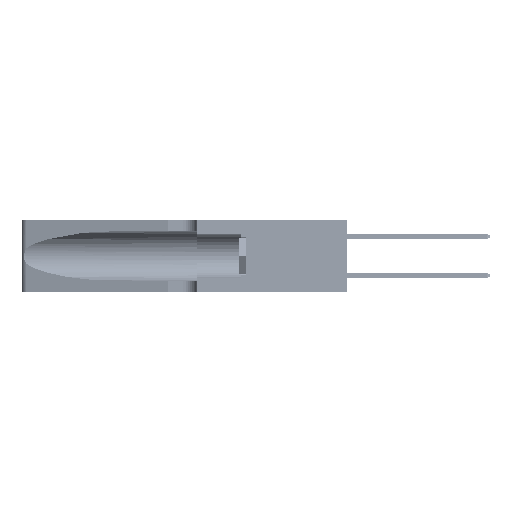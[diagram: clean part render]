
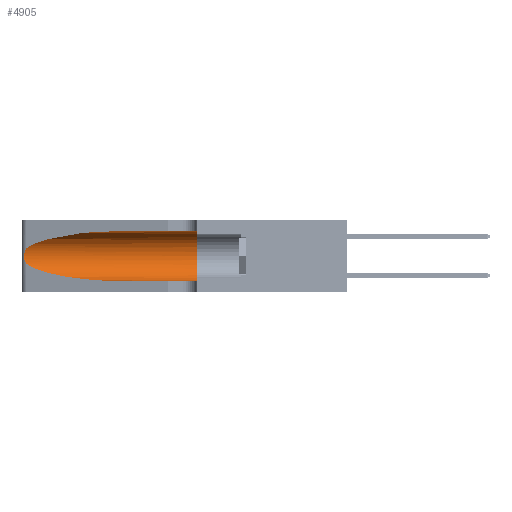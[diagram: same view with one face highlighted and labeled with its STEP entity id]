
A CAD part, left-side view. The second image highlights one B-rep face of the part: STEP entity #4905.
In plain terms, the highlighted cylindrical face has radius 3.308 mm (diameter 6.617 mm), a partial arc.
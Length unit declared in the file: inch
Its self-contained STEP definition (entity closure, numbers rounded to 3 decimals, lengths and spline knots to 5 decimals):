
#337 =( BOUNDED_CURVE ( )  B_SPLINE_CURVE ( 3, ( #11936, #41555, #20118, #29381 ),
 .UNSPECIFIED., .F., .F. ) 
 B_SPLINE_CURVE_WITH_KNOTS ( ( 4, 4 ),
 ( 3.44316, 4.71239 ),
 .UNSPECIFIED. ) 
 CURVE ( )  GEOMETRIC_REPRESENTATION_ITEM ( )  RATIONAL_B_SPLINE_CURVE ( ( 1., 0.87, 0.87, 1. ) ) 
 REPRESENTATION_ITEM ( '' )  );
#1661 = LINE ( 'NONE', #37860, #40006 ) ;
#2851 = CARTESIAN_POINT ( 'NONE',  ( 0.25639, 1.23184, 0.21858 ) ) ;
#2947 = EDGE_CURVE ( 'NONE', #52856, #15381, #337, .T. ) ;
#4281 = VERTEX_POINT ( 'NONE', #29657 ) ;
#4905 = ADVANCED_FACE ( 'NONE', ( #43117 ), #30594, .F. ) ;
#5707 = ORIENTED_EDGE ( 'NONE', *, *, #17141, .T. ) ;
#6196 = ORIENTED_EDGE ( 'NONE', *, *, #31475, .T. ) ;
#6332 = EDGE_CURVE ( 'NONE', #4281, #52856, #23085, .T. ) ;
#6570 = CARTESIAN_POINT ( 'NONE',  ( 0.25856, 1.23593, 0.16098 ) ) ;
#6740 = CARTESIAN_POINT ( 'NONE',  ( 0.25555, 1.22993, 0.14849 ) ) ;
#6777 = CARTESIAN_POINT ( 'NONE',  ( 0.1305, 0.72297, 0.05475 ) ) ;
#8695 = CARTESIAN_POINT ( 'NONE',  ( 0.1305, 0.72297, 0.31525 ) ) ;
#11936 = CARTESIAN_POINT ( 'NONE',  ( 0.25487, 1.22718, 0.14631 ) ) ;
#11962 = AXIS2_PLACEMENT_3D ( 'NONE', #54475, #29167, #32885 ) ;
#14701 = CARTESIAN_POINT ( 'NONE',  ( 0.26017, 1.23833, 0.17102 ) ) ;
#14808 = EDGE_LOOP ( 'NONE', ( #6196, #34730, #25363, #5707, #32238, #33674 ) ) ;
#15381 = VERTEX_POINT ( 'NONE', #6777 ) ;
#15561 = VERTEX_POINT ( 'NONE', #16351 ) ;
#15657 = DIRECTION ( 'NONE',  ( 0., 0., -1. ) ) ;
#16351 = CARTESIAN_POINT ( 'NONE',  ( 0.1305, 0.35, 0.05475 ) ) ;
#17141 = EDGE_CURVE ( 'NONE', #15381, #15561, #17456, .T. ) ;
#17456 = LINE ( 'NONE', #52339, #24165 ) ;
#19331 = CARTESIAN_POINT ( 'NONE',  ( 0.25789, 1.23486, 0.15765 ) ) ;
#20118 = CARTESIAN_POINT ( 'NONE',  ( 0.18966, 0.96281, 0.05475 ) ) ;
#22068 = VERTEX_POINT ( 'NONE', #8695 ) ;
#23085 = B_SPLINE_CURVE_WITH_KNOTS ( 'NONE', 3,
 ( #24001, #28256, #2851, #28069, #40047, #44654, #23451, #53013, #14701, #6570, #19331, #44309, #6740, #27713 ),
 .UNSPECIFIED., .F., .F.,
 ( 4, 2, 2, 2, 2, 2, 4 ),
 ( 0., 0.00027, 0.00053, 0.00107, 0.0016, 0.00187, 0.00214 ),
 .UNSPECIFIED. ) ;
#23451 = CARTESIAN_POINT ( 'NONE',  ( 0.26075, 1.23896, 0.19203 ) ) ;
#24001 = CARTESIAN_POINT ( 'NONE',  ( 0.25487, 1.22718, 0.22369 ) ) ;
#24165 = VECTOR ( 'NONE', #27052, 39.37008 ) ;
#24771 =( BOUNDED_CURVE ( )  B_SPLINE_CURVE ( 3, ( #42064, #46116, #51137, #33790 ),
 .UNSPECIFIED., .F., .F. ) 
 B_SPLINE_CURVE_WITH_KNOTS ( ( 4, 4 ),
 ( 1.5708, 2.84003 ),
 .UNSPECIFIED. ) 
 CURVE ( )  GEOMETRIC_REPRESENTATION_ITEM ( )  RATIONAL_B_SPLINE_CURVE ( ( 1., 0.87, 0.87, 1. ) ) 
 REPRESENTATION_ITEM ( '' )  );
#24961 = DIRECTION ( 'NONE',  ( 0., -1., 0. ) ) ;
#25363 = ORIENTED_EDGE ( 'NONE', *, *, #2947, .T. ) ;
#25509 = CARTESIAN_POINT ( 'NONE',  ( 0.25487, 1.22718, 0.14631 ) ) ;
#27052 = DIRECTION ( 'NONE',  ( 0., -1., 0. ) ) ;
#27515 = AXIS2_PLACEMENT_3D ( 'NONE', #45974, #24961, #15657 ) ;
#27713 = CARTESIAN_POINT ( 'NONE',  ( 0.25487, 1.22718, 0.14631 ) ) ;
#28069 = CARTESIAN_POINT ( 'NONE',  ( 0.25787, 1.23484, 0.2124 ) ) ;
#28256 = CARTESIAN_POINT ( 'NONE',  ( 0.25555, 1.22994, 0.2215 ) ) ;
#29167 = DIRECTION ( 'NONE',  ( 0., 1., 0. ) ) ;
#29204 = CARTESIAN_POINT ( 'NONE',  ( 0.1305, 0.35, 0.31525 ) ) ;
#29381 = CARTESIAN_POINT ( 'NONE',  ( 0.1305, 0.72297, 0.05475 ) ) ;
#29657 = CARTESIAN_POINT ( 'NONE',  ( 0.25487, 1.22718, 0.22369 ) ) ;
#30594 = CYLINDRICAL_SURFACE ( 'NONE', #27515, 0.13025 ) ;
#31238 = EDGE_CURVE ( 'NONE', #47429, #15561, #34085, .T. ) ;
#31475 = EDGE_CURVE ( 'NONE', #22068, #4281, #24771, .T. ) ;
#32238 = ORIENTED_EDGE ( 'NONE', *, *, #31238, .F. ) ;
#32885 = DIRECTION ( 'NONE',  ( 0., 0., 1. ) ) ;
#33674 = ORIENTED_EDGE ( 'NONE', *, *, #54036, .F. ) ;
#33790 = CARTESIAN_POINT ( 'NONE',  ( 0.25487, 1.22718, 0.22369 ) ) ;
#34085 = CIRCLE ( 'NONE', #11962, 0.13025 ) ;
#34730 = ORIENTED_EDGE ( 'NONE', *, *, #6332, .T. ) ;
#37860 = CARTESIAN_POINT ( 'NONE',  ( 0.1305, 1.61858, 0.31525 ) ) ;
#40006 = VECTOR ( 'NONE', #51363, 39.37008 ) ;
#40047 = CARTESIAN_POINT ( 'NONE',  ( 0.25854, 1.2359, 0.20912 ) ) ;
#41555 = CARTESIAN_POINT ( 'NONE',  ( 0.2373, 1.15595, 0.08982 ) ) ;
#42064 = CARTESIAN_POINT ( 'NONE',  ( 0.1305, 0.72297, 0.31525 ) ) ;
#43117 = FACE_OUTER_BOUND ( 'NONE', #14808, .T. ) ;
#44309 = CARTESIAN_POINT ( 'NONE',  ( 0.25639, 1.23186, 0.15144 ) ) ;
#44654 = CARTESIAN_POINT ( 'NONE',  ( 0.26018, 1.23835, 0.19895 ) ) ;
#45974 = CARTESIAN_POINT ( 'NONE',  ( 0.1305, 1.61858, 0.185 ) ) ;
#46116 = CARTESIAN_POINT ( 'NONE',  ( 0.18966, 0.96281, 0.31525 ) ) ;
#47429 = VERTEX_POINT ( 'NONE', #29204 ) ;
#51137 = CARTESIAN_POINT ( 'NONE',  ( 0.2373, 1.15595, 0.28018 ) ) ;
#51363 = DIRECTION ( 'NONE',  ( 0., -1., 0. ) ) ;
#52339 = CARTESIAN_POINT ( 'NONE',  ( 0.1305, 1.61858, 0.05475 ) ) ;
#52856 = VERTEX_POINT ( 'NONE', #25509 ) ;
#53013 = CARTESIAN_POINT ( 'NONE',  ( 0.26075, 1.23896, 0.178 ) ) ;
#54036 = EDGE_CURVE ( 'NONE', #22068, #47429, #1661, .T. ) ;
#54475 = CARTESIAN_POINT ( 'NONE',  ( 0.1305, 0.35, 0.185 ) ) ;
